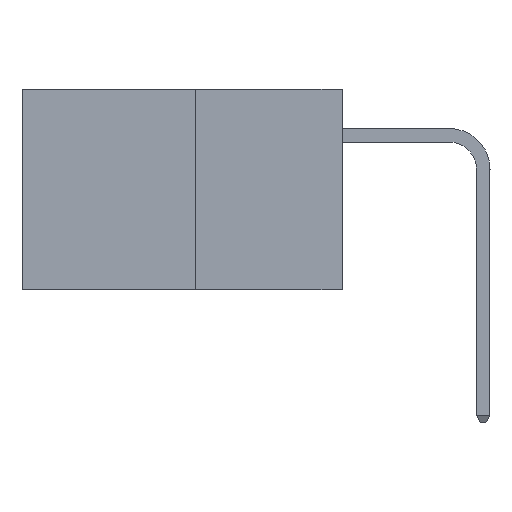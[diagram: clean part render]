
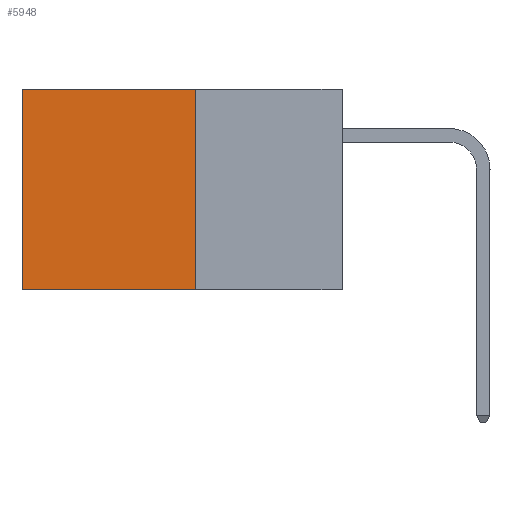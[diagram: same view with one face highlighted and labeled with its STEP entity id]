
A CAD part, left-side view. The second image highlights one B-rep face of the part: STEP entity #5948.
In plain terms, the highlighted planar face has unit normal (-1, 0, 0).
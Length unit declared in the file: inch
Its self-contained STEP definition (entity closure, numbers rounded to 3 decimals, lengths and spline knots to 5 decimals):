
#306 = CARTESIAN_POINT ( 'NONE',  ( 0.277, 0.27, -0.37 ) ) ;
#505 = ORIENTED_EDGE ( 'NONE', *, *, #12712, .F. ) ;
#2373 = EDGE_CURVE ( 'NONE', #5847, #9282, #7623, .T. ) ;
#2503 = VECTOR ( 'NONE', #16441, 39.37008 ) ;
#2526 = DIRECTION ( 'NONE',  ( 0., 0., -1. ) ) ;
#2651 = DIRECTION ( 'NONE',  ( 1., 0., 0. ) ) ;
#2763 = PLANE ( 'NONE',  #2887 ) ;
#2887 = AXIS2_PLACEMENT_3D ( 'NONE', #3705, #2651, #2526 ) ;
#3020 = CARTESIAN_POINT ( 'NONE',  ( 0.277, 0.27, -0.37 ) ) ;
#3198 = CARTESIAN_POINT ( 'NONE',  ( 0.277, 0.59, -0.37 ) ) ;
#3705 = CARTESIAN_POINT ( 'NONE',  ( 0.277, 0.27, -0.37 ) ) ;
#3779 = CARTESIAN_POINT ( 'NONE',  ( 0.277, 0.59, -0.37 ) ) ;
#3938 = VECTOR ( 'NONE', #7198, 39.37008 ) ;
#4236 = ORIENTED_EDGE ( 'NONE', *, *, #2373, .T. ) ;
#4788 = CARTESIAN_POINT ( 'NONE',  ( 0.277, 0.27, 0. ) ) ;
#4837 = DIRECTION ( 'NONE',  ( 0., 0., -1. ) ) ;
#5192 = DIRECTION ( 'NONE',  ( 0., 0., -1. ) ) ;
#5595 = VERTEX_POINT ( 'NONE', #3020 ) ;
#5847 = VERTEX_POINT ( 'NONE', #7492 ) ;
#5948 = ADVANCED_FACE ( 'NONE', ( #16734 ), #2763, .F. ) ;
#7198 = DIRECTION ( 'NONE',  ( 0., 1., 0. ) ) ;
#7351 = EDGE_LOOP ( 'NONE', ( #10295, #505, #17286, #4236 ) ) ;
#7492 = CARTESIAN_POINT ( 'NONE',  ( 0.277, 0.27, 0. ) ) ;
#7623 = LINE ( 'NONE', #4788, #3938 ) ;
#8388 = VERTEX_POINT ( 'NONE', #3779 ) ;
#9282 = VERTEX_POINT ( 'NONE', #11269 ) ;
#9674 = VECTOR ( 'NONE', #5192, 39.37008 ) ;
#10015 = EDGE_CURVE ( 'NONE', #9282, #8388, #10956, .T. ) ;
#10295 = ORIENTED_EDGE ( 'NONE', *, *, #10015, .T. ) ;
#10956 = LINE ( 'NONE', #3198, #14028 ) ;
#11269 = CARTESIAN_POINT ( 'NONE',  ( 0.277, 0.59, 0. ) ) ;
#12712 = EDGE_CURVE ( 'NONE', #5595, #8388, #13771, .T. ) ;
#13312 = CARTESIAN_POINT ( 'NONE',  ( 0.277, 0.27, -0.37 ) ) ;
#13771 = LINE ( 'NONE', #306, #2503 ) ;
#14028 = VECTOR ( 'NONE', #4837, 39.37008 ) ;
#16163 = LINE ( 'NONE', #13312, #9674 ) ;
#16441 = DIRECTION ( 'NONE',  ( 0., 1., 0. ) ) ;
#16734 = FACE_OUTER_BOUND ( 'NONE', #7351, .T. ) ;
#17286 = ORIENTED_EDGE ( 'NONE', *, *, #17301, .F. ) ;
#17301 = EDGE_CURVE ( 'NONE', #5847, #5595, #16163, .T. ) ;
